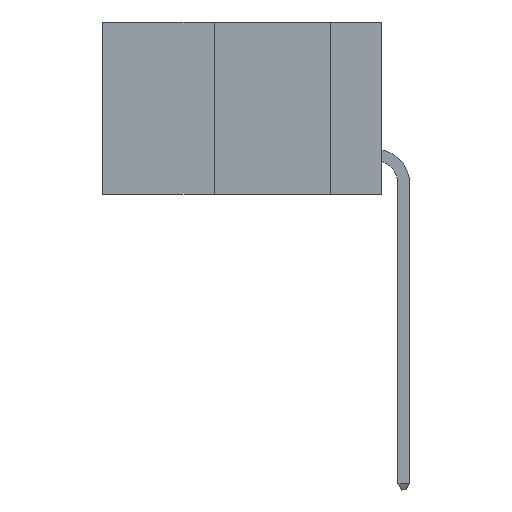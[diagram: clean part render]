
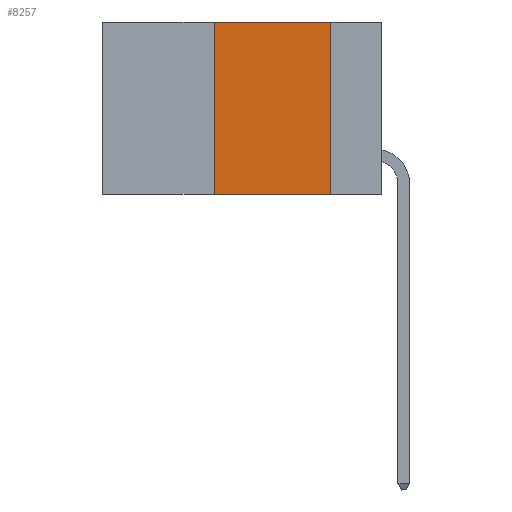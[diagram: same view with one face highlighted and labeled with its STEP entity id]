
A CAD part, left-side view. The second image highlights one B-rep face of the part: STEP entity #8257.
In plain terms, the highlighted planar face has unit normal (-1, 0, 0).
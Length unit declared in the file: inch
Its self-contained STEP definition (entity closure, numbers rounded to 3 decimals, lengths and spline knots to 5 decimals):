
#828 = DIRECTION ( 'NONE',  ( 0., -1., 0. ) ) ;
#850 = VERTEX_POINT ( 'NONE', #1602 ) ;
#1028 = ORIENTED_EDGE ( 'NONE', *, *, #4555, .T. ) ;
#1602 = CARTESIAN_POINT ( 'NONE',  ( 0., 0.36, -0.37 ) ) ;
#1734 = EDGE_CURVE ( 'NONE', #4658, #1974, #6293, .T. ) ;
#1974 = VERTEX_POINT ( 'NONE', #5319 ) ;
#2051 = FACE_OUTER_BOUND ( 'NONE', #3543, .T. ) ;
#2126 = LINE ( 'NONE', #11181, #10153 ) ;
#2336 = LINE ( 'NONE', #2394, #9788 ) ;
#2394 = CARTESIAN_POINT ( 'NONE',  ( 0., 0.6, 0. ) ) ;
#2440 = LINE ( 'NONE', #4927, #5349 ) ;
#3543 = EDGE_LOOP ( 'NONE', ( #4982, #7054, #4766, #1028 ) ) ;
#3827 = PLANE ( 'NONE',  #6431 ) ;
#4123 = EDGE_CURVE ( 'NONE', #850, #9342, #2126, .T. ) ;
#4555 = EDGE_CURVE ( 'NONE', #850, #1974, #2440, .T. ) ;
#4658 = VERTEX_POINT ( 'NONE', #5967 ) ;
#4766 = ORIENTED_EDGE ( 'NONE', *, *, #4123, .F. ) ;
#4815 = VECTOR ( 'NONE', #8107, 39.37008 ) ;
#4889 = DIRECTION ( 'NONE',  ( 0., -1., 0. ) ) ;
#4927 = CARTESIAN_POINT ( 'NONE',  ( 0., 0.6, -0.37 ) ) ;
#4982 = ORIENTED_EDGE ( 'NONE', *, *, #1734, .F. ) ;
#5319 = CARTESIAN_POINT ( 'NONE',  ( 0., 0.11, -0.37 ) ) ;
#5349 = VECTOR ( 'NONE', #4889, 39.37008 ) ;
#5540 = DIRECTION ( 'NONE',  ( 0., 0., -1. ) ) ;
#5909 = CARTESIAN_POINT ( 'NONE',  ( 0., 0.36, 0. ) ) ;
#5967 = CARTESIAN_POINT ( 'NONE',  ( 0., 0.11, 0. ) ) ;
#6293 = LINE ( 'NONE', #9942, #4815 ) ;
#6431 = AXIS2_PLACEMENT_3D ( 'NONE', #7486, #9411, #5540 ) ;
#7054 = ORIENTED_EDGE ( 'NONE', *, *, #8226, .F. ) ;
#7486 = CARTESIAN_POINT ( 'NONE',  ( 0., 0.6, 0. ) ) ;
#8107 = DIRECTION ( 'NONE',  ( 0., 0., -1. ) ) ;
#8226 = EDGE_CURVE ( 'NONE', #9342, #4658, #2336, .T. ) ;
#8257 = ADVANCED_FACE ( 'NONE', ( #2051 ), #3827, .F. ) ;
#9342 = VERTEX_POINT ( 'NONE', #5909 ) ;
#9411 = DIRECTION ( 'NONE',  ( 1., 0., 0. ) ) ;
#9538 = DIRECTION ( 'NONE',  ( 0., 0., 1. ) ) ;
#9788 = VECTOR ( 'NONE', #828, 39.37008 ) ;
#9942 = CARTESIAN_POINT ( 'NONE',  ( 0., 0.11, 0. ) ) ;
#10153 = VECTOR ( 'NONE', #9538, 39.37008 ) ;
#11181 = CARTESIAN_POINT ( 'NONE',  ( 0., 0.36, 0. ) ) ;
